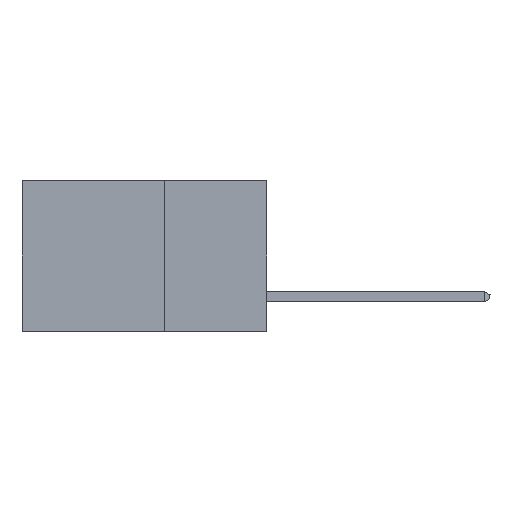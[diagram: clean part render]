
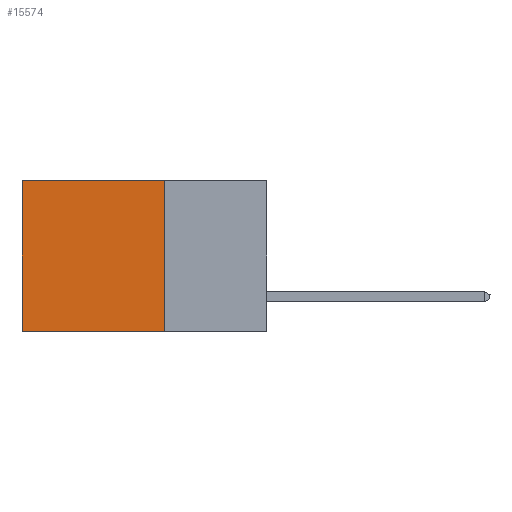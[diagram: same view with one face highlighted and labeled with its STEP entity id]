
A CAD part, left-side view. The second image highlights one B-rep face of the part: STEP entity #15574.
In plain terms, the highlighted planar face has unit normal (-1, 0, 0).
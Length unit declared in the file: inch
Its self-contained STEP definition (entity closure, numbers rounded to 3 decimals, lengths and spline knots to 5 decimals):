
#1514 = CARTESIAN_POINT ( 'NONE',  ( 0.2875, 0.6, 0. ) ) ;
#2312 = CARTESIAN_POINT ( 'NONE',  ( 0.2875, 0.25, 0. ) ) ;
#2319 = ORIENTED_EDGE ( 'NONE', *, *, #34610, .T. ) ;
#4533 = LINE ( 'NONE', #4989, #10446 ) ;
#4989 = CARTESIAN_POINT ( 'NONE',  ( 0.2875, 0.25, -0.37 ) ) ;
#5491 = ORIENTED_EDGE ( 'NONE', *, *, #31160, .T. ) ;
#7375 = VERTEX_POINT ( 'NONE', #30323 ) ;
#9389 = PLANE ( 'NONE',  #36960 ) ;
#9607 = DIRECTION ( 'NONE',  ( 0., 0., -1. ) ) ;
#9910 = CARTESIAN_POINT ( 'NONE',  ( 0.2875, 0.25, 0. ) ) ;
#10129 = VERTEX_POINT ( 'NONE', #1514 ) ;
#10446 = VECTOR ( 'NONE', #30355, 39.37008 ) ;
#12482 = CARTESIAN_POINT ( 'NONE',  ( 0.2875, 0.25, 0. ) ) ;
#15574 = ADVANCED_FACE ( 'NONE', ( #16956 ), #9389, .F. ) ;
#16105 = VERTEX_POINT ( 'NONE', #37999 ) ;
#16956 = FACE_OUTER_BOUND ( 'NONE', #28888, .T. ) ;
#20021 = VECTOR ( 'NONE', #38364, 39.37008 ) ;
#20267 = DIRECTION ( 'NONE',  ( 1., 0., 0. ) ) ;
#22008 = VERTEX_POINT ( 'NONE', #29938 ) ;
#22745 = LINE ( 'NONE', #26545, #43364 ) ;
#26545 = CARTESIAN_POINT ( 'NONE',  ( 0.2875, 0.6, 0. ) ) ;
#27923 = DIRECTION ( 'NONE',  ( 0., 1., 0. ) ) ;
#28205 = EDGE_CURVE ( 'NONE', #16105, #7375, #4533, .T. ) ;
#28888 = EDGE_LOOP ( 'NONE', ( #2319, #37440, #34465, #5491 ) ) ;
#29938 = CARTESIAN_POINT ( 'NONE',  ( 0.2875, 0.25, 0. ) ) ;
#30323 = CARTESIAN_POINT ( 'NONE',  ( 0.2875, 0.6, -0.37 ) ) ;
#30355 = DIRECTION ( 'NONE',  ( 0., 1., 0. ) ) ;
#31160 = EDGE_CURVE ( 'NONE', #22008, #10129, #35301, .T. ) ;
#34465 = ORIENTED_EDGE ( 'NONE', *, *, #37556, .F. ) ;
#34610 = EDGE_CURVE ( 'NONE', #10129, #7375, #22745, .T. ) ;
#34796 = LINE ( 'NONE', #2312, #20021 ) ;
#35301 = LINE ( 'NONE', #9910, #43281 ) ;
#36960 = AXIS2_PLACEMENT_3D ( 'NONE', #12482, #20267, #9607 ) ;
#37440 = ORIENTED_EDGE ( 'NONE', *, *, #28205, .F. ) ;
#37556 = EDGE_CURVE ( 'NONE', #22008, #16105, #34796, .T. ) ;
#37999 = CARTESIAN_POINT ( 'NONE',  ( 0.2875, 0.25, -0.37 ) ) ;
#38364 = DIRECTION ( 'NONE',  ( 0., 0., -1. ) ) ;
#41041 = DIRECTION ( 'NONE',  ( 0., 0., -1. ) ) ;
#43281 = VECTOR ( 'NONE', #27923, 39.37008 ) ;
#43364 = VECTOR ( 'NONE', #41041, 39.37008 ) ;
